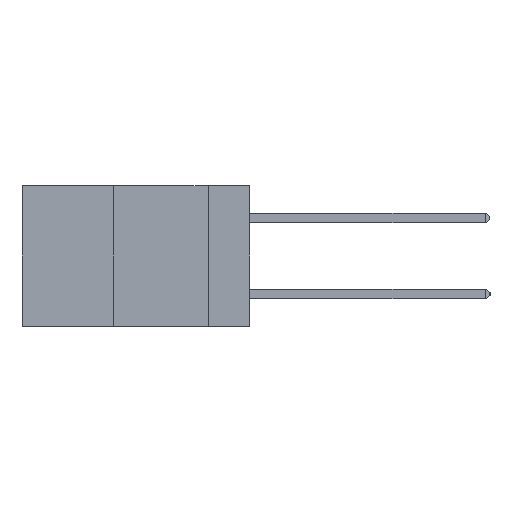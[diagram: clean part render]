
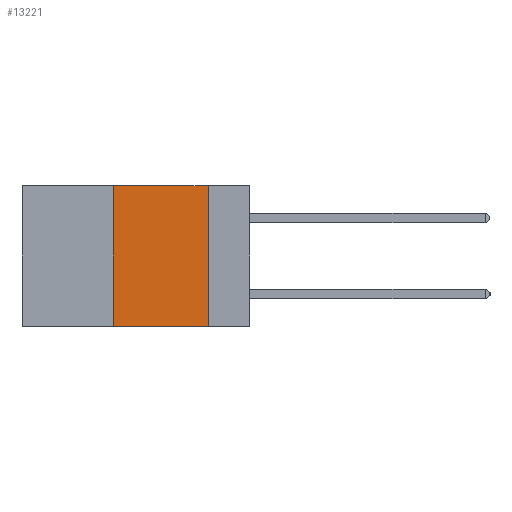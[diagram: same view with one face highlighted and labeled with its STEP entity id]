
A CAD part, left-side view. The second image highlights one B-rep face of the part: STEP entity #13221.
In plain terms, the highlighted planar face has unit normal (-1, 0, 0).
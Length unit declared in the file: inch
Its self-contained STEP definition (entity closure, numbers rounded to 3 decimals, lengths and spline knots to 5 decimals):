
#55 = EDGE_CURVE ( 'NONE', #5096, #10186, #13028, .T. ) ;
#737 = VECTOR ( 'NONE', #5248, 39.37008 ) ;
#1373 = EDGE_CURVE ( 'NONE', #13601, #2808, #12628, .T. ) ;
#1790 = CARTESIAN_POINT ( 'NONE',  ( 0., 0.6, 0. ) ) ;
#2179 = CARTESIAN_POINT ( 'NONE',  ( 0., 0.36, 0. ) ) ;
#2702 = CARTESIAN_POINT ( 'NONE',  ( 0., 0.6, 0. ) ) ;
#2808 = VERTEX_POINT ( 'NONE', #2179 ) ;
#3879 = DIRECTION ( 'NONE',  ( 0., 0., -1. ) ) ;
#4542 = CARTESIAN_POINT ( 'NONE',  ( 0., 0.36, -0.37 ) ) ;
#5096 = VERTEX_POINT ( 'NONE', #6650 ) ;
#5248 = DIRECTION ( 'NONE',  ( 0., 0., -1. ) ) ;
#5323 = DIRECTION ( 'NONE',  ( 0., -1., 0. ) ) ;
#5459 = VECTOR ( 'NONE', #5323, 39.37008 ) ;
#6141 = DIRECTION ( 'NONE',  ( 0., 0., 1. ) ) ;
#6650 = CARTESIAN_POINT ( 'NONE',  ( 0., 0.11, 0. ) ) ;
#6742 = FACE_OUTER_BOUND ( 'NONE', #12062, .T. ) ;
#6857 = EDGE_CURVE ( 'NONE', #13601, #10186, #7369, .T. ) ;
#6868 = CARTESIAN_POINT ( 'NONE',  ( 0., 0.36, 0. ) ) ;
#7369 = LINE ( 'NONE', #14539, #9649 ) ;
#7455 = EDGE_CURVE ( 'NONE', #2808, #5096, #12264, .T. ) ;
#9166 = CARTESIAN_POINT ( 'NONE',  ( 0., 0.11, 0. ) ) ;
#9646 = VECTOR ( 'NONE', #6141, 39.37008 ) ;
#9649 = VECTOR ( 'NONE', #13546, 39.37008 ) ;
#9660 = PLANE ( 'NONE',  #13812 ) ;
#9853 = ORIENTED_EDGE ( 'NONE', *, *, #55, .F. ) ;
#9870 = ORIENTED_EDGE ( 'NONE', *, *, #7455, .F. ) ;
#9959 = ORIENTED_EDGE ( 'NONE', *, *, #1373, .F. ) ;
#9971 = ORIENTED_EDGE ( 'NONE', *, *, #6857, .T. ) ;
#10186 = VERTEX_POINT ( 'NONE', #13064 ) ;
#10788 = DIRECTION ( 'NONE',  ( 1., 0., 0. ) ) ;
#12062 = EDGE_LOOP ( 'NONE', ( #9853, #9870, #9959, #9971 ) ) ;
#12264 = LINE ( 'NONE', #1790, #5459 ) ;
#12628 = LINE ( 'NONE', #6868, #9646 ) ;
#13028 = LINE ( 'NONE', #9166, #737 ) ;
#13064 = CARTESIAN_POINT ( 'NONE',  ( 0., 0.11, -0.37 ) ) ;
#13221 = ADVANCED_FACE ( 'NONE', ( #6742 ), #9660, .F. ) ;
#13546 = DIRECTION ( 'NONE',  ( 0., -1., 0. ) ) ;
#13601 = VERTEX_POINT ( 'NONE', #4542 ) ;
#13812 = AXIS2_PLACEMENT_3D ( 'NONE', #2702, #10788, #3879 ) ;
#14539 = CARTESIAN_POINT ( 'NONE',  ( 0., 0.6, -0.37 ) ) ;
